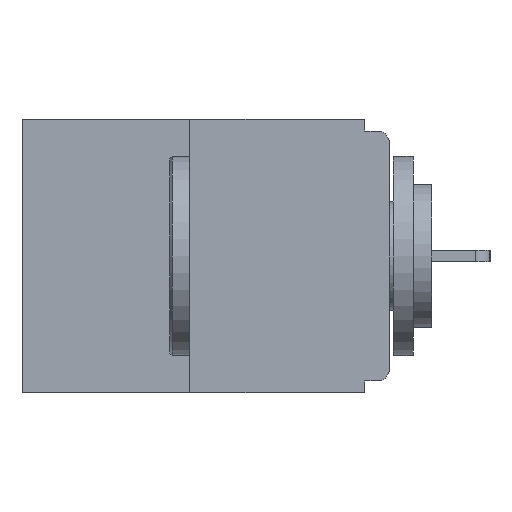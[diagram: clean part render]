
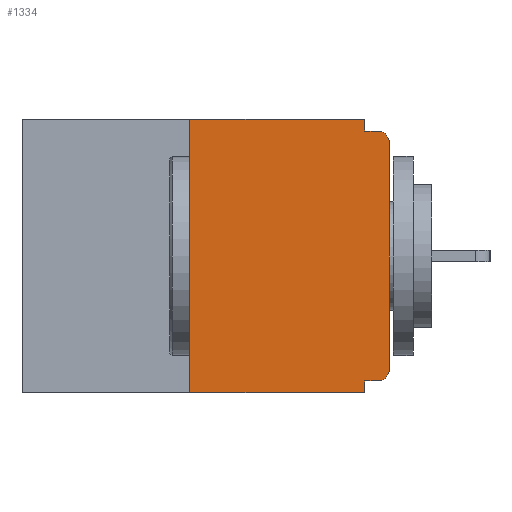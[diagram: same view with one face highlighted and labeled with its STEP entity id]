
A CAD part, left-side view. The second image highlights one B-rep face of the part: STEP entity #1334.
In plain terms, the highlighted planar face has unit normal (-1, 0, 0).
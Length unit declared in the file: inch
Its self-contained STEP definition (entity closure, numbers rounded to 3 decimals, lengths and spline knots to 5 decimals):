
#105 = LINE ( 'NONE', #1272, #17456 ) ;
#448 = AXIS2_PLACEMENT_3D ( 'NONE', #2956, #14713, #4706 ) ;
#982 = EDGE_CURVE ( 'NONE', #16685, #20397, #17148, .T. ) ;
#1272 = CARTESIAN_POINT ( 'NONE',  ( 0., 0.46, -0.343 ) ) ;
#1318 = VERTEX_POINT ( 'NONE', #12119 ) ;
#1334 = ADVANCED_FACE ( 'NONE', ( #15350 ), #11976, .F. ) ;
#1989 = CIRCLE ( 'NONE', #448, 0.015 ) ;
#2031 = DIRECTION ( 'NONE',  ( -1., 0., 0. ) ) ;
#2529 = CARTESIAN_POINT ( 'NONE',  ( 0., 0.25, 0. ) ) ;
#2956 = CARTESIAN_POINT ( 'NONE',  ( 0., 0.015, -0.03 ) ) ;
#3052 = LINE ( 'NONE', #20373, #11523 ) ;
#3473 = CARTESIAN_POINT ( 'NONE',  ( 0., 0.031, -0.343 ) ) ;
#3489 = AXIS2_PLACEMENT_3D ( 'NONE', #12165, #2031, #13822 ) ;
#3839 = VERTEX_POINT ( 'NONE', #19708 ) ;
#3840 = CARTESIAN_POINT ( 'NONE',  ( 0., 0.015, -0.328 ) ) ;
#4302 = DIRECTION ( 'NONE',  ( 0., 0., 1. ) ) ;
#4687 = VECTOR ( 'NONE', #4302, 39.37008 ) ;
#4696 = EDGE_LOOP ( 'NONE', ( #6072, #13912, #14948, #17270, #19360, #10337, #15287, #9786, #5184, #13585 ) ) ;
#4706 = DIRECTION ( 'NONE',  ( 0., 0., -1. ) ) ;
#4823 = VERTEX_POINT ( 'NONE', #5286 ) ;
#4851 = AXIS2_PLACEMENT_3D ( 'NONE', #17093, #12599, #12319 ) ;
#5184 = ORIENTED_EDGE ( 'NONE', *, *, #982, .F. ) ;
#5225 = LINE ( 'NONE', #2529, #4687 ) ;
#5286 = CARTESIAN_POINT ( 'NONE',  ( 0., 0.25, -0.343 ) ) ;
#5775 = CIRCLE ( 'NONE', #3489, 0.015 ) ;
#5974 = EDGE_CURVE ( 'NONE', #14439, #3839, #3052, .T. ) ;
#6072 = ORIENTED_EDGE ( 'NONE', *, *, #7938, .F. ) ;
#6292 = CARTESIAN_POINT ( 'NONE',  ( 0., 0.031, -0.015 ) ) ;
#6618 = CARTESIAN_POINT ( 'NONE',  ( 0., 0., -0.313 ) ) ;
#7731 = EDGE_CURVE ( 'NONE', #13358, #1318, #11743, .T. ) ;
#7938 = EDGE_CURVE ( 'NONE', #13431, #21103, #16334, .T. ) ;
#8339 = VECTOR ( 'NONE', #13552, 39.37008 ) ;
#9786 = ORIENTED_EDGE ( 'NONE', *, *, #17283, .T. ) ;
#10337 = ORIENTED_EDGE ( 'NONE', *, *, #17577, .T. ) ;
#11523 = VECTOR ( 'NONE', #20026, 39.37008 ) ;
#11603 = CARTESIAN_POINT ( 'NONE',  ( 0., 0.031, 0. ) ) ;
#11743 = LINE ( 'NONE', #20181, #19993 ) ;
#11976 = PLANE ( 'NONE',  #4851 ) ;
#12029 = CARTESIAN_POINT ( 'NONE',  ( 0., 0.031, -0.343 ) ) ;
#12119 = CARTESIAN_POINT ( 'NONE',  ( 0., 0.031, -0.328 ) ) ;
#12165 = CARTESIAN_POINT ( 'NONE',  ( 0., 0.015, -0.313 ) ) ;
#12319 = DIRECTION ( 'NONE',  ( 0., 0., -1. ) ) ;
#12480 = VECTOR ( 'NONE', #17266, 39.37008 ) ;
#12599 = DIRECTION ( 'NONE',  ( 1., 0., 0. ) ) ;
#13358 = VERTEX_POINT ( 'NONE', #3840 ) ;
#13431 = VERTEX_POINT ( 'NONE', #20655 ) ;
#13552 = DIRECTION ( 'NONE',  ( 0., -1., 0. ) ) ;
#13576 = CARTESIAN_POINT ( 'NONE',  ( 0., 0., -0.015 ) ) ;
#13585 = ORIENTED_EDGE ( 'NONE', *, *, #20620, .F. ) ;
#13822 = DIRECTION ( 'NONE',  ( 0., 0., -1. ) ) ;
#13912 = ORIENTED_EDGE ( 'NONE', *, *, #14791, .F. ) ;
#14356 = EDGE_CURVE ( 'NONE', #4823, #15693, #105, .T. ) ;
#14439 = VERTEX_POINT ( 'NONE', #6618 ) ;
#14516 = EDGE_CURVE ( 'NONE', #1318, #15693, #14892, .T. ) ;
#14713 = DIRECTION ( 'NONE',  ( -1., 0., 0. ) ) ;
#14791 = EDGE_CURVE ( 'NONE', #4823, #13431, #5225, .T. ) ;
#14892 = LINE ( 'NONE', #3473, #19282 ) ;
#14948 = ORIENTED_EDGE ( 'NONE', *, *, #14356, .T. ) ;
#15206 = DIRECTION ( 'NONE',  ( 0., 0., -1. ) ) ;
#15287 = ORIENTED_EDGE ( 'NONE', *, *, #5974, .T. ) ;
#15350 = FACE_OUTER_BOUND ( 'NONE', #4696, .T. ) ;
#15693 = VERTEX_POINT ( 'NONE', #12029 ) ;
#16334 = LINE ( 'NONE', #17312, #12480 ) ;
#16406 = DIRECTION ( 'NONE',  ( 0., -1., 0. ) ) ;
#16685 = VERTEX_POINT ( 'NONE', #6292 ) ;
#17093 = CARTESIAN_POINT ( 'NONE',  ( 0., 0.46, 0. ) ) ;
#17148 = LINE ( 'NONE', #13576, #8339 ) ;
#17266 = DIRECTION ( 'NONE',  ( 0., -1., 0. ) ) ;
#17270 = ORIENTED_EDGE ( 'NONE', *, *, #14516, .F. ) ;
#17283 = EDGE_CURVE ( 'NONE', #3839, #20397, #1989, .T. ) ;
#17312 = CARTESIAN_POINT ( 'NONE',  ( 0., 0.46, 0. ) ) ;
#17456 = VECTOR ( 'NONE', #16406, 39.37008 ) ;
#17561 = CARTESIAN_POINT ( 'NONE',  ( 0., 0.015, -0.015 ) ) ;
#17577 = EDGE_CURVE ( 'NONE', #13358, #14439, #5775, .T. ) ;
#17685 = CARTESIAN_POINT ( 'NONE',  ( 0., 0.031, 0. ) ) ;
#18139 = DIRECTION ( 'NONE',  ( 0., 0., -1. ) ) ;
#19282 = VECTOR ( 'NONE', #15206, 39.37008 ) ;
#19360 = ORIENTED_EDGE ( 'NONE', *, *, #7731, .F. ) ;
#19652 = LINE ( 'NONE', #11603, #20679 ) ;
#19708 = CARTESIAN_POINT ( 'NONE',  ( 0., 0., -0.03 ) ) ;
#19993 = VECTOR ( 'NONE', #20175, 39.37008 ) ;
#20026 = DIRECTION ( 'NONE',  ( 0., 0., 1. ) ) ;
#20175 = DIRECTION ( 'NONE',  ( 0., 1., 0. ) ) ;
#20181 = CARTESIAN_POINT ( 'NONE',  ( 0., 0., -0.328 ) ) ;
#20373 = CARTESIAN_POINT ( 'NONE',  ( 0., 0., 0. ) ) ;
#20397 = VERTEX_POINT ( 'NONE', #17561 ) ;
#20620 = EDGE_CURVE ( 'NONE', #21103, #16685, #19652, .T. ) ;
#20655 = CARTESIAN_POINT ( 'NONE',  ( 0., 0.25, 0. ) ) ;
#20679 = VECTOR ( 'NONE', #18139, 39.37008 ) ;
#21103 = VERTEX_POINT ( 'NONE', #17685 ) ;
